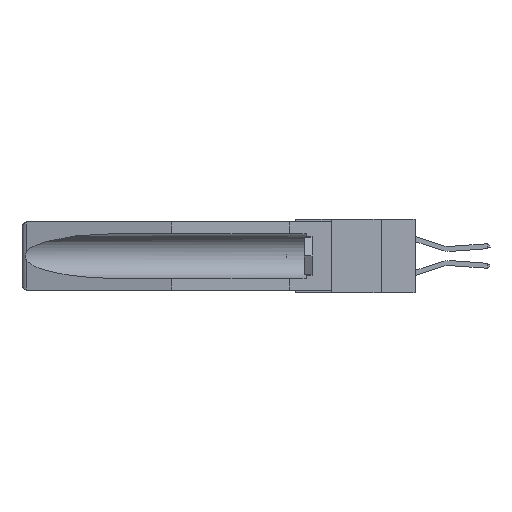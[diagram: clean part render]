
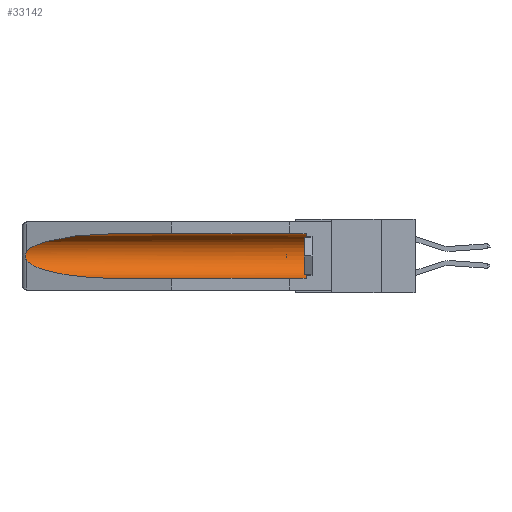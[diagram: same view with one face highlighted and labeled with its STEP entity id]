
A CAD part, left-side view. The second image highlights one B-rep face of the part: STEP entity #33142.
In plain terms, the highlighted cylindrical face has radius 2.857 mm (diameter 5.715 mm), a partial arc.
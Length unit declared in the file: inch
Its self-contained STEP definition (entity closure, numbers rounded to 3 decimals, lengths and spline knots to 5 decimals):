
#230 = B_SPLINE_CURVE_WITH_KNOTS ( 'NONE', 3,
 ( #20390, #3742, #9572, #23175, #9680, #15390, #28979, #6658, #34306, #26435 ),
 .UNSPECIFIED., .F., .F.,
 ( 4, 2, 2, 2, 4 ),
 ( 0., 0.00029, 0.00058, 0.00087, 0.00117 ),
 .UNSPECIFIED. ) ;
#893 = CARTESIAN_POINT ( 'NONE',  ( 0.155, -0.30754, -0.1715 ) ) ;
#927 = CARTESIAN_POINT ( 'NONE',  ( 0.155, 1.07973, -0.284 ) ) ;
#1056 = DIRECTION ( 'NONE',  ( 0., 1., 0. ) ) ;
#1917 = CARTESIAN_POINT ( 'NONE',  ( 0.155, 0.126, -0.059 ) ) ;
#3705 = DIRECTION ( 'NONE',  ( 0., 1., 0. ) ) ;
#3742 = CARTESIAN_POINT ( 'NONE',  ( 0.26597, 1.52961, -0.15275 ) ) ;
#4159 = VERTEX_POINT ( 'NONE', #32564 ) ;
#4964 = VERTEX_POINT ( 'NONE', #927 ) ;
#5836 = EDGE_CURVE ( 'NONE', #6697, #4964, #13148, .T. ) ;
#6273 = CARTESIAN_POINT ( 'NONE',  ( 0.21114, 1.30732, -0.284 ) ) ;
#6658 = CARTESIAN_POINT ( 'NONE',  ( 0.26655, 1.53094, -0.18657 ) ) ;
#6697 = VERTEX_POINT ( 'NONE', #8992 ) ;
#8424 = CIRCLE ( 'NONE', #31470, 0.1125 ) ;
#8543 = ORIENTED_EDGE ( 'NONE', *, *, #27367, .T. ) ;
#8992 = CARTESIAN_POINT ( 'NONE',  ( 0.26537, 1.52718, -0.19328 ) ) ;
#8996 = AXIS2_PLACEMENT_3D ( 'NONE', #893, #3705, #23141 ) ;
#9296 = CARTESIAN_POINT ( 'NONE',  ( 0.26537, 1.52718, -0.19328 ) ) ;
#9572 = CARTESIAN_POINT ( 'NONE',  ( 0.26654, 1.53092, -0.15636 ) ) ;
#9680 = CARTESIAN_POINT ( 'NONE',  ( 0.2675, 1.53308, -0.16763 ) ) ;
#10545 = CARTESIAN_POINT ( 'NONE',  ( 0.155, -0.30754, -0.059 ) ) ;
#10651 = VERTEX_POINT ( 'NONE', #25208 ) ;
#11701 = CARTESIAN_POINT ( 'NONE',  ( 0.155, 0.126, -0.1715 ) ) ;
#11755 = CARTESIAN_POINT ( 'NONE',  ( 0.155, -0.30754, -0.284 ) ) ;
#11828 = VECTOR ( 'NONE', #1056, 39.37008 ) ;
#13106 = CARTESIAN_POINT ( 'NONE',  ( 0.155, 0.126, -0.284 ) ) ;
#13148 =( BOUNDED_CURVE ( )  B_SPLINE_CURVE ( 3, ( #9296, #23152, #6273, #25423 ),
 .UNSPECIFIED., .F., .F. ) 
 B_SPLINE_CURVE_WITH_KNOTS ( ( 4, 4 ),
 ( 0.1948, 1.5708 ),
 .UNSPECIFIED. ) 
 CURVE ( )  GEOMETRIC_REPRESENTATION_ITEM ( )  RATIONAL_B_SPLINE_CURVE ( ( 1., 0.848, 0.848, 1. ) ) 
 REPRESENTATION_ITEM ( '' )  );
#13927 = EDGE_CURVE ( 'NONE', #16255, #4964, #16581, .T. ) ;
#15390 = CARTESIAN_POINT ( 'NONE',  ( 0.2675, 1.53308, -0.17534 ) ) ;
#16255 = VERTEX_POINT ( 'NONE', #13106 ) ;
#16581 = LINE ( 'NONE', #11755, #11828 ) ;
#16907 =( BOUNDED_CURVE ( )  B_SPLINE_CURVE ( 3, ( #22861, #25731, #25606, #31182 ),
 .UNSPECIFIED., .F., .F. ) 
 B_SPLINE_CURVE_WITH_KNOTS ( ( 4, 4 ),
 ( 4.71239, 6.08839 ),
 .UNSPECIFIED. ) 
 CURVE ( )  GEOMETRIC_REPRESENTATION_ITEM ( )  RATIONAL_B_SPLINE_CURVE ( ( 1., 0.848, 0.848, 1. ) ) 
 REPRESENTATION_ITEM ( '' )  );
#17172 = EDGE_CURVE ( 'NONE', #16255, #34904, #8424, .T. ) ;
#18975 = EDGE_CURVE ( 'NONE', #4159, #6697, #230, .T. ) ;
#20390 = CARTESIAN_POINT ( 'NONE',  ( 0.26537, 1.52718, -0.14972 ) ) ;
#21299 = CYLINDRICAL_SURFACE ( 'NONE', #8996, 0.1125 ) ;
#22861 = CARTESIAN_POINT ( 'NONE',  ( 0.155, 1.07973, -0.059 ) ) ;
#23009 = DIRECTION ( 'NONE',  ( 0., -1., 0. ) ) ;
#23141 = DIRECTION ( 'NONE',  ( 0., 0., 1. ) ) ;
#23152 = CARTESIAN_POINT ( 'NONE',  ( 0.25451, 1.48313, -0.24835 ) ) ;
#23175 = CARTESIAN_POINT ( 'NONE',  ( 0.2673, 1.5327, -0.16383 ) ) ;
#25208 = CARTESIAN_POINT ( 'NONE',  ( 0.155, 1.07973, -0.059 ) ) ;
#25423 = CARTESIAN_POINT ( 'NONE',  ( 0.155, 1.07973, -0.284 ) ) ;
#25606 = CARTESIAN_POINT ( 'NONE',  ( 0.25451, 1.48313, -0.09465 ) ) ;
#25731 = CARTESIAN_POINT ( 'NONE',  ( 0.21114, 1.30732, -0.059 ) ) ;
#25883 = DIRECTION ( 'NONE',  ( 0., 0., 1. ) ) ;
#26435 = CARTESIAN_POINT ( 'NONE',  ( 0.26537, 1.52718, -0.19328 ) ) ;
#26782 = ORIENTED_EDGE ( 'NONE', *, *, #18975, .T. ) ;
#26925 = FACE_OUTER_BOUND ( 'NONE', #29187, .T. ) ;
#27040 = DIRECTION ( 'NONE',  ( 0., 1., 0. ) ) ;
#27367 = EDGE_CURVE ( 'NONE', #34904, #10651, #28950, .T. ) ;
#28689 = EDGE_CURVE ( 'NONE', #10651, #4159, #16907, .T. ) ;
#28950 = LINE ( 'NONE', #10545, #29361 ) ;
#28979 = CARTESIAN_POINT ( 'NONE',  ( 0.2673, 1.53269, -0.17917 ) ) ;
#29187 = EDGE_LOOP ( 'NONE', ( #34014, #26782, #35747, #34093, #34972, #8543 ) ) ;
#29361 = VECTOR ( 'NONE', #27040, 39.37008 ) ;
#31182 = CARTESIAN_POINT ( 'NONE',  ( 0.26537, 1.52718, -0.14972 ) ) ;
#31470 = AXIS2_PLACEMENT_3D ( 'NONE', #11701, #23009, #25883 ) ;
#32564 = CARTESIAN_POINT ( 'NONE',  ( 0.26537, 1.52718, -0.14972 ) ) ;
#33142 = ADVANCED_FACE ( 'NONE', ( #26925 ), #21299, .F. ) ;
#34014 = ORIENTED_EDGE ( 'NONE', *, *, #28689, .T. ) ;
#34093 = ORIENTED_EDGE ( 'NONE', *, *, #13927, .F. ) ;
#34306 = CARTESIAN_POINT ( 'NONE',  ( 0.26597, 1.5296, -0.19026 ) ) ;
#34904 = VERTEX_POINT ( 'NONE', #1917 ) ;
#34972 = ORIENTED_EDGE ( 'NONE', *, *, #17172, .T. ) ;
#35747 = ORIENTED_EDGE ( 'NONE', *, *, #5836, .T. ) ;
